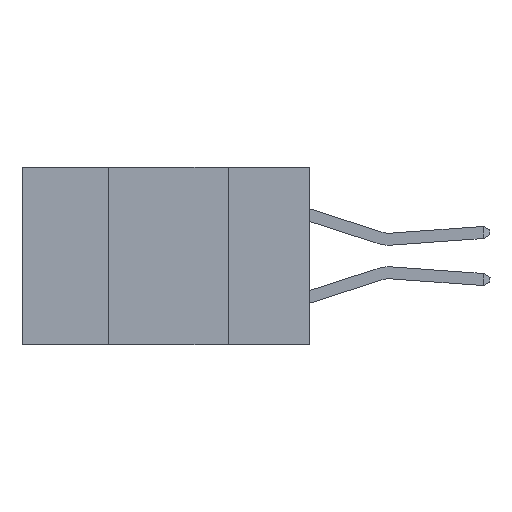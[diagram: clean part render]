
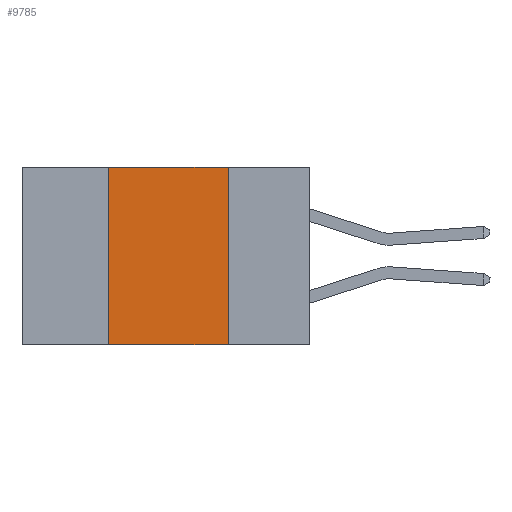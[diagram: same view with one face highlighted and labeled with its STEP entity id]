
A CAD part, left-side view. The second image highlights one B-rep face of the part: STEP entity #9785.
In plain terms, the highlighted planar face has unit normal (-1, 0, 0).
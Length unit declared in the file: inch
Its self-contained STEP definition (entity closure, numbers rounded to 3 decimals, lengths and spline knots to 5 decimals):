
#459 = CARTESIAN_POINT ( 'NONE',  ( 0., 0.6, -0.37 ) ) ;
#768 = CARTESIAN_POINT ( 'NONE',  ( 0., 0.17, 0. ) ) ;
#799 = LINE ( 'NONE', #459, #11162 ) ;
#1520 = DIRECTION ( 'NONE',  ( 0., 0., 1. ) ) ;
#1595 = VERTEX_POINT ( 'NONE', #14952 ) ;
#1715 = LINE ( 'NONE', #14507, #18714 ) ;
#3088 = DIRECTION ( 'NONE',  ( 0., 0., -1. ) ) ;
#4761 = ORIENTED_EDGE ( 'NONE', *, *, #9698, .T. ) ;
#4838 = FACE_OUTER_BOUND ( 'NONE', #7357, .T. ) ;
#5703 = VERTEX_POINT ( 'NONE', #7159 ) ;
#6683 = VECTOR ( 'NONE', #7512, 39.37008 ) ;
#7159 = CARTESIAN_POINT ( 'NONE',  ( 0., 0.42, -0.37 ) ) ;
#7271 = DIRECTION ( 'NONE',  ( 1., 0., 0. ) ) ;
#7357 = EDGE_LOOP ( 'NONE', ( #16091, #10204, #25536, #4761 ) ) ;
#7512 = DIRECTION ( 'NONE',  ( 0., -1., 0. ) ) ;
#8076 = LINE ( 'NONE', #22902, #24401 ) ;
#9698 = EDGE_CURVE ( 'NONE', #5703, #1595, #799, .T. ) ;
#9785 = ADVANCED_FACE ( 'NONE', ( #4838 ), #15700, .F. ) ;
#10111 = AXIS2_PLACEMENT_3D ( 'NONE', #19789, #7271, #3088 ) ;
#10204 = ORIENTED_EDGE ( 'NONE', *, *, #18716, .F. ) ;
#11162 = VECTOR ( 'NONE', #23603, 39.37008 ) ;
#12324 = LINE ( 'NONE', #24579, #6683 ) ;
#14507 = CARTESIAN_POINT ( 'NONE',  ( 0., 0.17, 0. ) ) ;
#14786 = DIRECTION ( 'NONE',  ( 0., 0., -1. ) ) ;
#14952 = CARTESIAN_POINT ( 'NONE',  ( 0., 0.17, -0.37 ) ) ;
#15700 = PLANE ( 'NONE',  #10111 ) ;
#16091 = ORIENTED_EDGE ( 'NONE', *, *, #22143, .F. ) ;
#16193 = CARTESIAN_POINT ( 'NONE',  ( 0., 0.42, 0. ) ) ;
#18418 = EDGE_CURVE ( 'NONE', #5703, #26240, #8076, .T. ) ;
#18714 = VECTOR ( 'NONE', #14786, 39.37008 ) ;
#18716 = EDGE_CURVE ( 'NONE', #26240, #18909, #12324, .T. ) ;
#18909 = VERTEX_POINT ( 'NONE', #768 ) ;
#19789 = CARTESIAN_POINT ( 'NONE',  ( 0., 0.6, 0. ) ) ;
#22143 = EDGE_CURVE ( 'NONE', #18909, #1595, #1715, .T. ) ;
#22902 = CARTESIAN_POINT ( 'NONE',  ( 0., 0.42, 0. ) ) ;
#23603 = DIRECTION ( 'NONE',  ( 0., -1., 0. ) ) ;
#24401 = VECTOR ( 'NONE', #1520, 39.37008 ) ;
#24579 = CARTESIAN_POINT ( 'NONE',  ( 0., 0.6, 0. ) ) ;
#25536 = ORIENTED_EDGE ( 'NONE', *, *, #18418, .F. ) ;
#26240 = VERTEX_POINT ( 'NONE', #16193 ) ;
